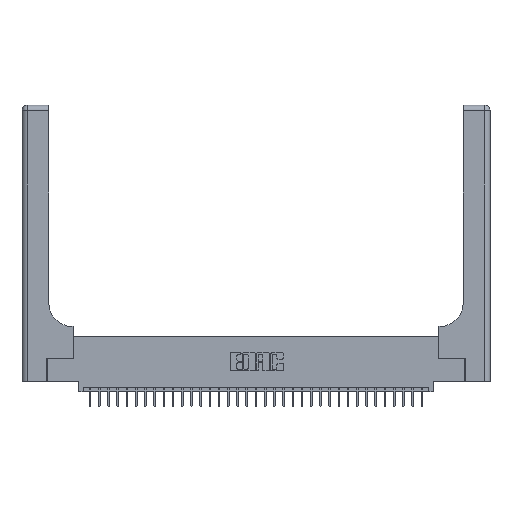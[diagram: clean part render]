
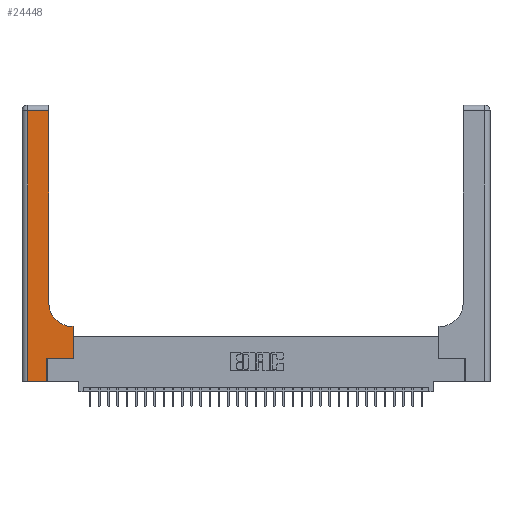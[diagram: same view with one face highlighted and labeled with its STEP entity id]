
A CAD part, top view. The second image highlights one B-rep face of the part: STEP entity #24448.
In plain terms, the highlighted planar face has unit normal (0, 0, 1).
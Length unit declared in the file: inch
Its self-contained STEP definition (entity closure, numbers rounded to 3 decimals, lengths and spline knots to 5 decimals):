
#1377 = CARTESIAN_POINT ( 'NONE',  ( 0.269, 0.25, 0.37 ) ) ;
#2322 = VERTEX_POINT ( 'NONE', #34083 ) ;
#2733 = DIRECTION ( 'NONE',  ( -1., 0., 0. ) ) ;
#3228 = DIRECTION ( 'NONE',  ( 0., 1., 0. ) ) ;
#3345 = CARTESIAN_POINT ( 'NONE',  ( 0.269, 0., 0.37 ) ) ;
#3798 = LINE ( 'NONE', #32003, #15742 ) ;
#4781 = LINE ( 'NONE', #24166, #17072 ) ;
#6356 = AXIS2_PLACEMENT_3D ( 'NONE', #29405, #32277, #2733 ) ;
#6854 = VERTEX_POINT ( 'NONE', #1377 ) ;
#7441 = CARTESIAN_POINT ( 'NONE',  ( 0.06, 0., 0.37 ) ) ;
#7993 = CARTESIAN_POINT ( 'NONE',  ( 0.06, 2.94, 0.37 ) ) ;
#8311 = EDGE_LOOP ( 'NONE', ( #28873, #26232, #22123, #33820, #32370, #14993, #31939, #19812, #33769 ) ) ;
#8415 = EDGE_CURVE ( 'NONE', #6854, #26801, #32826, .T. ) ;
#8574 = CARTESIAN_POINT ( 'NONE',  ( 0.2915, 0.85, 0.37 ) ) ;
#9509 = LINE ( 'NONE', #3345, #33274 ) ;
#10676 = EDGE_CURVE ( 'NONE', #2322, #16750, #21759, .T. ) ;
#10735 = LINE ( 'NONE', #19016, #24682 ) ;
#10744 = CARTESIAN_POINT ( 'NONE',  ( 0.06, 3., 0.37 ) ) ;
#10768 = CARTESIAN_POINT ( 'NONE',  ( 0.2915, 0.6, 0.37 ) ) ;
#10877 = DIRECTION ( 'NONE',  ( -1., 0., 0. ) ) ;
#10918 = DIRECTION ( 'NONE',  ( 0., 1., 0. ) ) ;
#11315 = EDGE_CURVE ( 'NONE', #12959, #30507, #3798, .T. ) ;
#11783 = CARTESIAN_POINT ( 'NONE',  ( 0., 0., 0.37 ) ) ;
#12959 = VERTEX_POINT ( 'NONE', #20495 ) ;
#13140 = DIRECTION ( 'NONE',  ( -1., 0., 0. ) ) ;
#13254 = DIRECTION ( 'NONE',  ( 0., -1., 0. ) ) ;
#14993 = ORIENTED_EDGE ( 'NONE', *, *, #8415, .T. ) ;
#15742 = VECTOR ( 'NONE', #13140, 39.37008 ) ;
#15916 = DIRECTION ( 'NONE',  ( 1., 0., 0. ) ) ;
#16122 = DIRECTION ( 'NONE',  ( 0., 1., 0. ) ) ;
#16676 = CARTESIAN_POINT ( 'NONE',  ( 0.269, 0., 0.37 ) ) ;
#16740 = DIRECTION ( 'NONE',  ( 1., 0., 0. ) ) ;
#16750 = VERTEX_POINT ( 'NONE', #8574 ) ;
#16880 = CARTESIAN_POINT ( 'NONE',  ( 0.5585, 0.25, 0.37 ) ) ;
#17072 = VECTOR ( 'NONE', #16122, 39.37008 ) ;
#17377 = LINE ( 'NONE', #11783, #28865 ) ;
#18929 = LINE ( 'NONE', #10768, #21046 ) ;
#19016 = CARTESIAN_POINT ( 'NONE',  ( 0.5585, 0.25, 0.37 ) ) ;
#19205 = VECTOR ( 'NONE', #13254, 39.37008 ) ;
#19812 = ORIENTED_EDGE ( 'NONE', *, *, #32661, .T. ) ;
#20056 = FACE_OUTER_BOUND ( 'NONE', #8311, .T. ) ;
#20495 = CARTESIAN_POINT ( 'NONE',  ( 0.2915, 2.94, 0.37 ) ) ;
#21046 = VECTOR ( 'NONE', #10877, 39.37008 ) ;
#21759 = CIRCLE ( 'NONE', #34366, 0.25 ) ;
#22123 = ORIENTED_EDGE ( 'NONE', *, *, #29834, .T. ) ;
#22750 = EDGE_CURVE ( 'NONE', #35030, #6854, #9509, .T. ) ;
#22983 = VERTEX_POINT ( 'NONE', #7441 ) ;
#24166 = CARTESIAN_POINT ( 'NONE',  ( 0.2915, 3., 0.37 ) ) ;
#24448 = ADVANCED_FACE ( 'NONE', ( #20056 ), #32499, .F. ) ;
#24668 = EDGE_CURVE ( 'NONE', #22983, #35030, #17377, .T. ) ;
#24682 = VECTOR ( 'NONE', #10918, 39.37008 ) ;
#26232 = ORIENTED_EDGE ( 'NONE', *, *, #11315, .T. ) ;
#26801 = VERTEX_POINT ( 'NONE', #16880 ) ;
#28017 = DIRECTION ( 'NONE',  ( 1., 0., 0. ) ) ;
#28342 = CARTESIAN_POINT ( 'NONE',  ( 0.269, 0.25, 0.37 ) ) ;
#28865 = VECTOR ( 'NONE', #28017, 39.37008 ) ;
#28873 = ORIENTED_EDGE ( 'NONE', *, *, #29847, .T. ) ;
#29405 = CARTESIAN_POINT ( 'NONE',  ( 0., 3., 0.37 ) ) ;
#29834 = EDGE_CURVE ( 'NONE', #30507, #22983, #33632, .T. ) ;
#29847 = EDGE_CURVE ( 'NONE', #16750, #12959, #4781, .T. ) ;
#30264 = DIRECTION ( 'NONE',  ( 0., 0., -1. ) ) ;
#30507 = VERTEX_POINT ( 'NONE', #7993 ) ;
#31121 = VECTOR ( 'NONE', #15916, 39.37008 ) ;
#31939 = ORIENTED_EDGE ( 'NONE', *, *, #33779, .T. ) ;
#32003 = CARTESIAN_POINT ( 'NONE',  ( 0., 2.94, 0.37 ) ) ;
#32277 = DIRECTION ( 'NONE',  ( 0., 0., -1. ) ) ;
#32370 = ORIENTED_EDGE ( 'NONE', *, *, #22750, .T. ) ;
#32499 = PLANE ( 'NONE',  #6356 ) ;
#32661 = EDGE_CURVE ( 'NONE', #32808, #2322, #18929, .T. ) ;
#32808 = VERTEX_POINT ( 'NONE', #33747 ) ;
#32826 = LINE ( 'NONE', #28342, #31121 ) ;
#33230 = CARTESIAN_POINT ( 'NONE',  ( 0.5415, 0.85, 0.37 ) ) ;
#33274 = VECTOR ( 'NONE', #3228, 39.37008 ) ;
#33632 = LINE ( 'NONE', #10744, #19205 ) ;
#33747 = CARTESIAN_POINT ( 'NONE',  ( 0.5585, 0.6, 0.37 ) ) ;
#33769 = ORIENTED_EDGE ( 'NONE', *, *, #10676, .T. ) ;
#33779 = EDGE_CURVE ( 'NONE', #26801, #32808, #10735, .T. ) ;
#33820 = ORIENTED_EDGE ( 'NONE', *, *, #24668, .T. ) ;
#34083 = CARTESIAN_POINT ( 'NONE',  ( 0.5415, 0.6, 0.37 ) ) ;
#34366 = AXIS2_PLACEMENT_3D ( 'NONE', #33230, #30264, #16740 ) ;
#35030 = VERTEX_POINT ( 'NONE', #16676 ) ;
